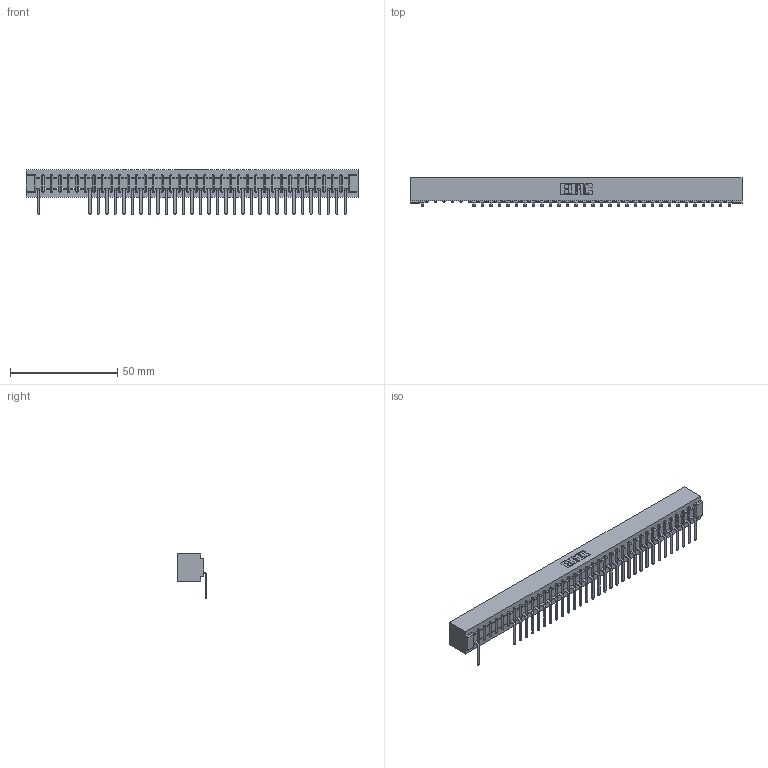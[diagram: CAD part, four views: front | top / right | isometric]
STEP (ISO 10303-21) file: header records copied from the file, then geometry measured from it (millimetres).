
FILE_DESCRIPTION (( 'STEP AP203' ), '1' );
FILE_NAME ('357-037-557-101.STEP', '2018-08-10T08:09:35', ( '' ), ( '' ), 'SwSTEP 2.0', 'SolidWorks 2016', '' );
FILE_SCHEMA (( 'CONFIG_CONTROL_DESIGN' ));
Length unit declared in the file: inch
Products named in the file (3): 307 Part_No Mounting Lugs; 307-290-002_557; 357-037-557-101
Assembly tree (33 placements, depth 2):
  357-037-557-101
    307 Part_No Mounting Lugs
    307-290-002_557  x32
Bounding box: 154.48 x 13.32 x 20.66 mm (x, y, z)
Volume: 16993.8 mm3; surface area: 21241.9 mm2
Topology: 33 solids, 33 shells, 2744 faces, 8427 edges, 5514 vertices
Faces by surface type: plane 1630, cylinder 1038, sphere 76
Entity records: 32752 total; most frequent: CARTESIAN_POINT 5547, ORIENTED_EDGE 5542, DIRECTION 5385, EDGE_CURVE 2771, LINE 2121, VECTOR 2121, VERTEX_POINT 1794, AXIS2_PLACEMENT_3D 1632
